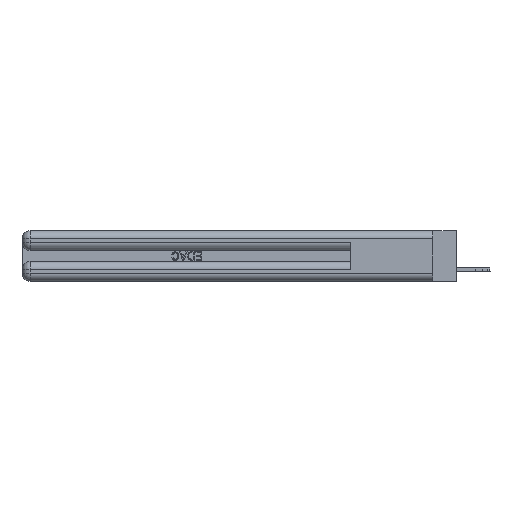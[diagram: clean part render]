
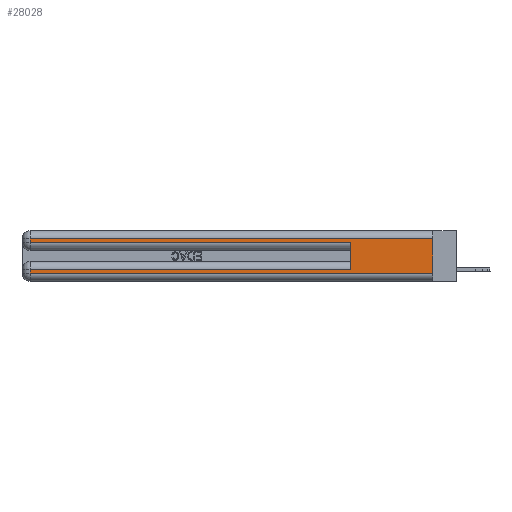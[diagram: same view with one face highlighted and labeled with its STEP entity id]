
A CAD part, left-side view. The second image highlights one B-rep face of the part: STEP entity #28028.
In plain terms, the highlighted planar face has unit normal (-1, 0, 0).
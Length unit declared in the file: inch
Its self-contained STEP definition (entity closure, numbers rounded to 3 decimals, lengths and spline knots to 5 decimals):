
#1426 = VERTEX_POINT ( 'NONE', #19529 ) ;
#1479 = EDGE_CURVE ( 'NONE', #28006, #28038, #16368, .T. ) ;
#1647 = EDGE_CURVE ( 'NONE', #26181, #36893, #32076, .T. ) ;
#2686 = VECTOR ( 'NONE', #37706, 39.37008 ) ;
#3723 = LINE ( 'NONE', #23273, #20903 ) ;
#4360 = CARTESIAN_POINT ( 'NONE',  ( 0., 0., 0.085 ) ) ;
#4513 = VECTOR ( 'NONE', #10207, 39.37008 ) ;
#5122 = DIRECTION ( 'NONE',  ( 0., 0., -1. ) ) ;
#6762 = CARTESIAN_POINT ( 'NONE',  ( 0., 0., 0.31 ) ) ;
#7151 = DIRECTION ( 'NONE',  ( 0., 1., 0. ) ) ;
#7311 = VERTEX_POINT ( 'NONE', #26204 ) ;
#7383 = CARTESIAN_POINT ( 'NONE',  ( 0., 0., 0.285 ) ) ;
#7484 = PLANE ( 'NONE',  #32863 ) ;
#8266 = VECTOR ( 'NONE', #11155, 39.37008 ) ;
#9776 = CARTESIAN_POINT ( 'NONE',  ( 0., 2.94, 0.37 ) ) ;
#9927 = EDGE_CURVE ( 'NONE', #7311, #26181, #19865, .T. ) ;
#10013 = CARTESIAN_POINT ( 'NONE',  ( 0., 2.94, 0.31 ) ) ;
#10150 = VECTOR ( 'NONE', #31294, 39.37008 ) ;
#10207 = DIRECTION ( 'NONE',  ( 0., -1., 0. ) ) ;
#10474 = DIRECTION ( 'NONE',  ( 0., -1., 0. ) ) ;
#11155 = DIRECTION ( 'NONE',  ( 0., 1., 0. ) ) ;
#12210 = EDGE_CURVE ( 'NONE', #28038, #1426, #24631, .T. ) ;
#12701 = VECTOR ( 'NONE', #22752, 39.37008 ) ;
#13471 = EDGE_CURVE ( 'NONE', #7311, #18837, #37812, .T. ) ;
#14476 = DIRECTION ( 'NONE',  ( 0., 0., 1. ) ) ;
#16368 = LINE ( 'NONE', #4360, #8266 ) ;
#17444 = CARTESIAN_POINT ( 'NONE',  ( 0., 0.6, 0.285 ) ) ;
#17862 = LINE ( 'NONE', #34219, #4513 ) ;
#18837 = VERTEX_POINT ( 'NONE', #30676 ) ;
#18908 = VECTOR ( 'NONE', #7151, 39.37008 ) ;
#19524 = ORIENTED_EDGE ( 'NONE', *, *, #12210, .T. ) ;
#19529 = CARTESIAN_POINT ( 'NONE',  ( 0., 2.94, 0.06 ) ) ;
#19829 = EDGE_CURVE ( 'NONE', #28006, #19836, #3723, .T. ) ;
#19836 = VERTEX_POINT ( 'NONE', #17444 ) ;
#19865 = LINE ( 'NONE', #6762, #18908 ) ;
#20058 = ORIENTED_EDGE ( 'NONE', *, *, #1479, .T. ) ;
#20284 = CARTESIAN_POINT ( 'NONE',  ( 0., 0., 0.37 ) ) ;
#20790 = ORIENTED_EDGE ( 'NONE', *, *, #13471, .F. ) ;
#20903 = VECTOR ( 'NONE', #14476, 39.37008 ) ;
#22081 = VECTOR ( 'NONE', #10474, 39.37008 ) ;
#22752 = DIRECTION ( 'NONE',  ( 0., 0., -1. ) ) ;
#23234 = CARTESIAN_POINT ( 'NONE',  ( 0., 2.94, 0.285 ) ) ;
#23273 = CARTESIAN_POINT ( 'NONE',  ( 0., 0.6, 0.145 ) ) ;
#24547 = ORIENTED_EDGE ( 'NONE', *, *, #19829, .F. ) ;
#24631 = LINE ( 'NONE', #37060, #12701 ) ;
#26109 = CARTESIAN_POINT ( 'NONE',  ( 0., 0.6, 0.085 ) ) ;
#26181 = VERTEX_POINT ( 'NONE', #10013 ) ;
#26204 = CARTESIAN_POINT ( 'NONE',  ( 0., 0., 0.31 ) ) ;
#28006 = VERTEX_POINT ( 'NONE', #26109 ) ;
#28028 = ADVANCED_FACE ( 'NONE', ( #29323 ), #7484, .F. ) ;
#28038 = VERTEX_POINT ( 'NONE', #38718 ) ;
#28075 = ORIENTED_EDGE ( 'NONE', *, *, #1647, .T. ) ;
#29313 = DIRECTION ( 'NONE',  ( 1., 0., 0. ) ) ;
#29323 = FACE_OUTER_BOUND ( 'NONE', #38252, .T. ) ;
#30242 = ORIENTED_EDGE ( 'NONE', *, *, #36787, .T. ) ;
#30615 = ORIENTED_EDGE ( 'NONE', *, *, #9927, .T. ) ;
#30676 = CARTESIAN_POINT ( 'NONE',  ( 0., 0., 0.06 ) ) ;
#31294 = DIRECTION ( 'NONE',  ( 0., 0., -1. ) ) ;
#32076 = LINE ( 'NONE', #9776, #10150 ) ;
#32863 = AXIS2_PLACEMENT_3D ( 'NONE', #20284, #29313, #5122 ) ;
#34219 = CARTESIAN_POINT ( 'NONE',  ( 0., 0., 0.06 ) ) ;
#34922 = LINE ( 'NONE', #7383, #22081 ) ;
#35816 = ORIENTED_EDGE ( 'NONE', *, *, #36758, .T. ) ;
#36758 = EDGE_CURVE ( 'NONE', #1426, #18837, #17862, .T. ) ;
#36787 = EDGE_CURVE ( 'NONE', #36893, #19836, #34922, .T. ) ;
#36893 = VERTEX_POINT ( 'NONE', #23234 ) ;
#37060 = CARTESIAN_POINT ( 'NONE',  ( 0., 2.94, 0.37 ) ) ;
#37575 = CARTESIAN_POINT ( 'NONE',  ( 0., 0., 0.37 ) ) ;
#37706 = DIRECTION ( 'NONE',  ( 0., 0., -1. ) ) ;
#37812 = LINE ( 'NONE', #37575, #2686 ) ;
#38252 = EDGE_LOOP ( 'NONE', ( #20790, #30615, #28075, #30242, #24547, #20058, #19524, #35816 ) ) ;
#38718 = CARTESIAN_POINT ( 'NONE',  ( 0., 2.94, 0.085 ) ) ;
